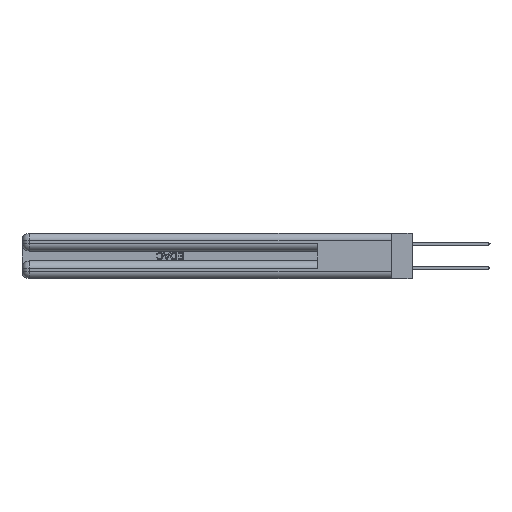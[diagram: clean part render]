
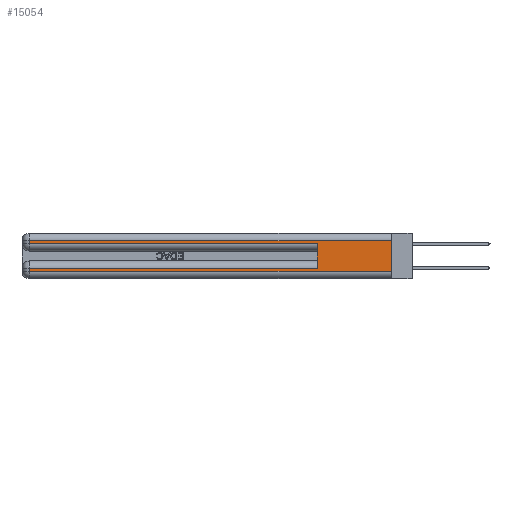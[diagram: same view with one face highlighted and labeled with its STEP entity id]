
A CAD part, left-side view. The second image highlights one B-rep face of the part: STEP entity #15054.
In plain terms, the highlighted planar face has unit normal (-1, 0, 0).
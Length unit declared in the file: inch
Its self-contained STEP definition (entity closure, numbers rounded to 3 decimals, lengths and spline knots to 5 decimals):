
#619 = DIRECTION ( 'NONE',  ( 1., 0., 0. ) ) ;
#1337 = CARTESIAN_POINT ( 'NONE',  ( 0., 2.94, 0.06 ) ) ;
#1415 = VECTOR ( 'NONE', #33366, 39.37008 ) ;
#1462 = EDGE_CURVE ( 'NONE', #24239, #30625, #33810, .T. ) ;
#2000 = VECTOR ( 'NONE', #47837, 39.37008 ) ;
#2508 = CARTESIAN_POINT ( 'NONE',  ( 0., 2.94, 0.31 ) ) ;
#2533 = EDGE_CURVE ( 'NONE', #22582, #38635, #45125, .T. ) ;
#3028 = VERTEX_POINT ( 'NONE', #34097 ) ;
#4377 = DIRECTION ( 'NONE',  ( 0., 0., -1. ) ) ;
#4558 = PLANE ( 'NONE',  #14674 ) ;
#5886 = DIRECTION ( 'NONE',  ( 0., 0., -1. ) ) ;
#6070 = CARTESIAN_POINT ( 'NONE',  ( 0., 2.94, 0.37 ) ) ;
#6823 = CARTESIAN_POINT ( 'NONE',  ( 0., 0., 0.31 ) ) ;
#9644 = VERTEX_POINT ( 'NONE', #6823 ) ;
#10366 = VERTEX_POINT ( 'NONE', #27167 ) ;
#11645 = ORIENTED_EDGE ( 'NONE', *, *, #1462, .T. ) ;
#11867 = LINE ( 'NONE', #39887, #44268 ) ;
#12527 = VECTOR ( 'NONE', #38656, 39.37008 ) ;
#13225 = EDGE_CURVE ( 'NONE', #9644, #3028, #49219, .T. ) ;
#14199 = DIRECTION ( 'NONE',  ( 0., 0., 1. ) ) ;
#14285 = ORIENTED_EDGE ( 'NONE', *, *, #39077, .T. ) ;
#14674 = AXIS2_PLACEMENT_3D ( 'NONE', #39382, #619, #4377 ) ;
#14893 = EDGE_CURVE ( 'NONE', #9644, #24239, #23815, .T. ) ;
#15004 = LINE ( 'NONE', #34726, #12527 ) ;
#15054 = ADVANCED_FACE ( 'NONE', ( #48964 ), #4558, .F. ) ;
#16694 = LINE ( 'NONE', #17137, #48435 ) ;
#17137 = CARTESIAN_POINT ( 'NONE',  ( 0., 0., 0.285 ) ) ;
#17463 = ORIENTED_EDGE ( 'NONE', *, *, #26061, .T. ) ;
#19559 = DIRECTION ( 'NONE',  ( 0., 1., 0. ) ) ;
#20171 = ORIENTED_EDGE ( 'NONE', *, *, #2533, .F. ) ;
#20425 = VERTEX_POINT ( 'NONE', #1337 ) ;
#22490 = CARTESIAN_POINT ( 'NONE',  ( 0., 2.94, 0.285 ) ) ;
#22582 = VERTEX_POINT ( 'NONE', #42004 ) ;
#23815 = LINE ( 'NONE', #42980, #30567 ) ;
#24239 = VERTEX_POINT ( 'NONE', #2508 ) ;
#26061 = EDGE_CURVE ( 'NONE', #22582, #10366, #15004, .T. ) ;
#27002 = LINE ( 'NONE', #32078, #2000 ) ;
#27167 = CARTESIAN_POINT ( 'NONE',  ( 0., 2.94, 0.085 ) ) ;
#28399 = DIRECTION ( 'NONE',  ( 0., -1., 0. ) ) ;
#28752 = ORIENTED_EDGE ( 'NONE', *, *, #14893, .T. ) ;
#30567 = VECTOR ( 'NONE', #19559, 39.37008 ) ;
#30625 = VERTEX_POINT ( 'NONE', #22490 ) ;
#30675 = EDGE_LOOP ( 'NONE', ( #48472, #28752, #11645, #43293, #20171, #17463, #14285, #40921 ) ) ;
#32078 = CARTESIAN_POINT ( 'NONE',  ( 0., 2.94, 0.37 ) ) ;
#33366 = DIRECTION ( 'NONE',  ( 0., 0., -1. ) ) ;
#33810 = LINE ( 'NONE', #6070, #1415 ) ;
#34097 = CARTESIAN_POINT ( 'NONE',  ( 0., 0., 0.06 ) ) ;
#34726 = CARTESIAN_POINT ( 'NONE',  ( 0., 0., 0.085 ) ) ;
#35720 = VECTOR ( 'NONE', #5886, 39.37008 ) ;
#38485 = EDGE_CURVE ( 'NONE', #30625, #38635, #16694, .T. ) ;
#38635 = VERTEX_POINT ( 'NONE', #45855 ) ;
#38656 = DIRECTION ( 'NONE',  ( 0., 1., 0. ) ) ;
#39077 = EDGE_CURVE ( 'NONE', #10366, #20425, #27002, .T. ) ;
#39382 = CARTESIAN_POINT ( 'NONE',  ( 0., 0., 0.37 ) ) ;
#39887 = CARTESIAN_POINT ( 'NONE',  ( 0., 0., 0.06 ) ) ;
#40710 = DIRECTION ( 'NONE',  ( 0., -1., 0. ) ) ;
#40921 = ORIENTED_EDGE ( 'NONE', *, *, #48272, .T. ) ;
#42004 = CARTESIAN_POINT ( 'NONE',  ( 0., 0.6, 0.085 ) ) ;
#42980 = CARTESIAN_POINT ( 'NONE',  ( 0., 0., 0.31 ) ) ;
#43293 = ORIENTED_EDGE ( 'NONE', *, *, #38485, .T. ) ;
#44268 = VECTOR ( 'NONE', #28399, 39.37008 ) ;
#44953 = CARTESIAN_POINT ( 'NONE',  ( 0., 0.6, 0.145 ) ) ;
#45125 = LINE ( 'NONE', #44953, #48821 ) ;
#45855 = CARTESIAN_POINT ( 'NONE',  ( 0., 0.6, 0.285 ) ) ;
#47837 = DIRECTION ( 'NONE',  ( 0., 0., -1. ) ) ;
#48272 = EDGE_CURVE ( 'NONE', #20425, #3028, #11867, .T. ) ;
#48435 = VECTOR ( 'NONE', #40710, 39.37008 ) ;
#48472 = ORIENTED_EDGE ( 'NONE', *, *, #13225, .F. ) ;
#48767 = CARTESIAN_POINT ( 'NONE',  ( 0., 0., 0.37 ) ) ;
#48821 = VECTOR ( 'NONE', #14199, 39.37008 ) ;
#48964 = FACE_OUTER_BOUND ( 'NONE', #30675, .T. ) ;
#49219 = LINE ( 'NONE', #48767, #35720 ) ;
